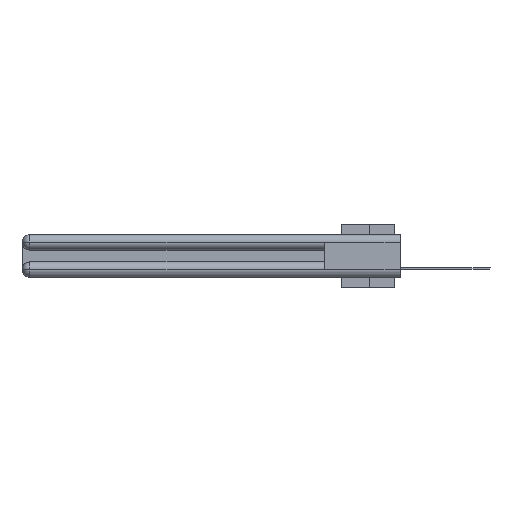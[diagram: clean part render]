
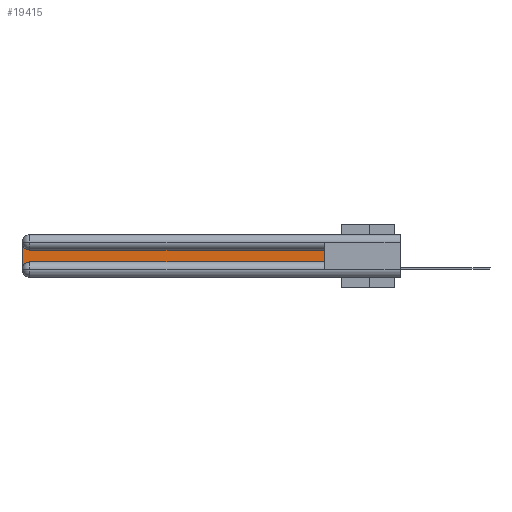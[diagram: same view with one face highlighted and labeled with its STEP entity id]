
A CAD part, left-side view. The second image highlights one B-rep face of the part: STEP entity #19415.
In plain terms, the highlighted planar face has unit normal (-1, 0, 0).
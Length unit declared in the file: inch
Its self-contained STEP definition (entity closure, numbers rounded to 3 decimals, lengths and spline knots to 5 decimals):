
#753 = DIRECTION ( 'NONE',  ( 1., 0., 0. ) ) ;
#1376 = CARTESIAN_POINT ( 'NONE',  ( 0.075, 0.6, -0.2175 ) ) ;
#2547 = VECTOR ( 'NONE', #27380, 39.37008 ) ;
#2666 = VERTEX_POINT ( 'NONE', #13049 ) ;
#2988 = AXIS2_PLACEMENT_3D ( 'NONE', #14015, #21938, #5967 ) ;
#3301 = EDGE_LOOP ( 'NONE', ( #29945, #8259, #12584, #8452, #29169, #31630 ) ) ;
#4091 = VERTEX_POINT ( 'NONE', #24311 ) ;
#4418 = CARTESIAN_POINT ( 'NONE',  ( 0.075, 3., -0.0625 ) ) ;
#4645 = LINE ( 'NONE', #20140, #31180 ) ;
#5967 = DIRECTION ( 'NONE',  ( 0., 0., -1. ) ) ;
#6212 = DIRECTION ( 'NONE',  ( 0., 0., -1. ) ) ;
#6509 = EDGE_CURVE ( 'NONE', #8685, #4091, #26319, .T. ) ;
#8259 = ORIENTED_EDGE ( 'NONE', *, *, #25544, .T. ) ;
#8452 = ORIENTED_EDGE ( 'NONE', *, *, #34514, .T. ) ;
#8685 = VERTEX_POINT ( 'NONE', #1376 ) ;
#8986 = EDGE_CURVE ( 'NONE', #28440, #8685, #4645, .T. ) ;
#10258 = CIRCLE ( 'NONE', #32402, 0.06 ) ;
#12115 = CARTESIAN_POINT ( 'NONE',  ( 0.075, 2.94, -0.2175 ) ) ;
#12584 = ORIENTED_EDGE ( 'NONE', *, *, #26848, .T. ) ;
#13049 = CARTESIAN_POINT ( 'NONE',  ( 0.075, 2.94, -0.1225 ) ) ;
#13710 = AXIS2_PLACEMENT_3D ( 'NONE', #30624, #22404, #6212 ) ;
#13723 = CARTESIAN_POINT ( 'NONE',  ( 0.075, 3., -0.2175 ) ) ;
#14015 = CARTESIAN_POINT ( 'NONE',  ( 0.075, 2.94, -0.2775 ) ) ;
#14385 = PLANE ( 'NONE',  #13710 ) ;
#17280 = DIRECTION ( 'NONE',  ( 0., 1., 0. ) ) ;
#19415 = ADVANCED_FACE ( 'NONE', ( #22990 ), #14385, .F. ) ;
#20092 = CARTESIAN_POINT ( 'NONE',  ( 0.075, 3., -0.2775 ) ) ;
#20140 = CARTESIAN_POINT ( 'NONE',  ( 0.075, 0.6, -0.2175 ) ) ;
#20384 = VERTEX_POINT ( 'NONE', #4418 ) ;
#20872 = VECTOR ( 'NONE', #17280, 39.37008 ) ;
#20928 = CIRCLE ( 'NONE', #2988, 0.06 ) ;
#21695 = DIRECTION ( 'NONE',  ( 0., 0., 1. ) ) ;
#21938 = DIRECTION ( 'NONE',  ( 1., 0., 0. ) ) ;
#22404 = DIRECTION ( 'NONE',  ( 1., 0., 0. ) ) ;
#22990 = FACE_OUTER_BOUND ( 'NONE', #3301, .T. ) ;
#23803 = VECTOR ( 'NONE', #21695, 39.37008 ) ;
#24311 = CARTESIAN_POINT ( 'NONE',  ( 0.075, 0.6, -0.1225 ) ) ;
#25170 = CARTESIAN_POINT ( 'NONE',  ( 0.075, 0.6, -0.1225 ) ) ;
#25544 = EDGE_CURVE ( 'NONE', #2666, #20384, #10258, .T. ) ;
#26319 = LINE ( 'NONE', #34954, #23803 ) ;
#26848 = EDGE_CURVE ( 'NONE', #20384, #31408, #29121, .T. ) ;
#27380 = DIRECTION ( 'NONE',  ( 0., 0., -1. ) ) ;
#27680 = CARTESIAN_POINT ( 'NONE',  ( 0.075, 2.94, -0.0625 ) ) ;
#27789 = DIRECTION ( 'NONE',  ( 0., 0., -1. ) ) ;
#28333 = DIRECTION ( 'NONE',  ( 0., -1., 0. ) ) ;
#28440 = VERTEX_POINT ( 'NONE', #12115 ) ;
#28952 = EDGE_CURVE ( 'NONE', #4091, #2666, #31784, .T. ) ;
#29121 = LINE ( 'NONE', #13723, #2547 ) ;
#29169 = ORIENTED_EDGE ( 'NONE', *, *, #8986, .T. ) ;
#29945 = ORIENTED_EDGE ( 'NONE', *, *, #28952, .T. ) ;
#30624 = CARTESIAN_POINT ( 'NONE',  ( 0.075, 3., -0.1225 ) ) ;
#31180 = VECTOR ( 'NONE', #28333, 39.37008 ) ;
#31408 = VERTEX_POINT ( 'NONE', #20092 ) ;
#31630 = ORIENTED_EDGE ( 'NONE', *, *, #6509, .T. ) ;
#31784 = LINE ( 'NONE', #25170, #20872 ) ;
#32402 = AXIS2_PLACEMENT_3D ( 'NONE', #27680, #753, #27789 ) ;
#34514 = EDGE_CURVE ( 'NONE', #31408, #28440, #20928, .T. ) ;
#34954 = CARTESIAN_POINT ( 'NONE',  ( 0.075, 0.6, -0.2175 ) ) ;
